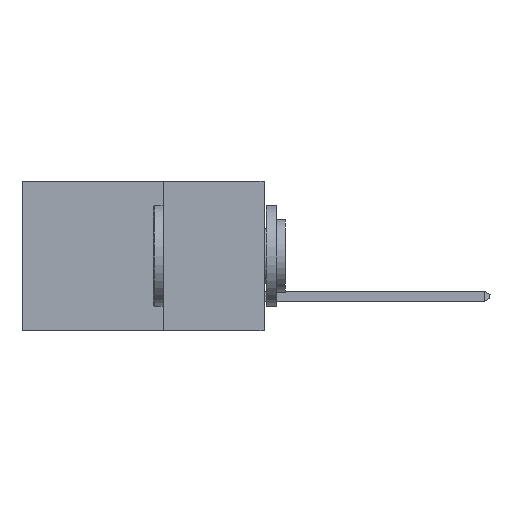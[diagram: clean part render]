
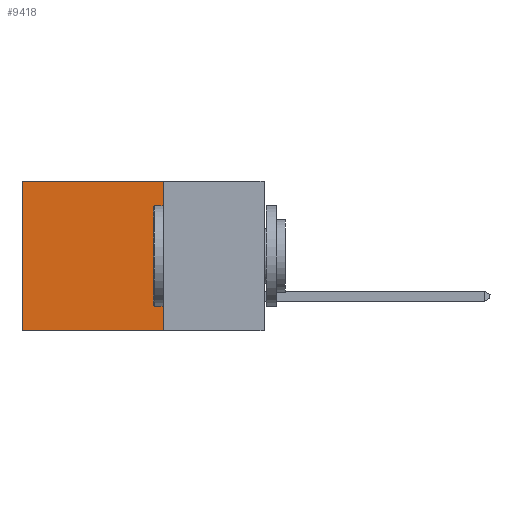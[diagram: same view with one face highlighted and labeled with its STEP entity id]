
A CAD part, left-side view. The second image highlights one B-rep face of the part: STEP entity #9418.
In plain terms, the highlighted planar face has unit normal (-1, 0, 0).
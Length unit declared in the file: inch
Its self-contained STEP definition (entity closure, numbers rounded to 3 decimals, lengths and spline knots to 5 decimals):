
#198 = LINE ( 'NONE', #7642, #2643 ) ;
#1241 = ORIENTED_EDGE ( 'NONE', *, *, #16333, .T. ) ;
#2643 = VECTOR ( 'NONE', #11825, 39.37008 ) ;
#2667 = DIRECTION ( 'NONE',  ( 1., 0., 0. ) ) ;
#2674 = CARTESIAN_POINT ( 'NONE',  ( 0.2615, 0.25, 0. ) ) ;
#3452 = CARTESIAN_POINT ( 'NONE',  ( 0.2615, 0.25, -0.37 ) ) ;
#3565 = DIRECTION ( 'NONE',  ( 0., 0., -1. ) ) ;
#3681 = VERTEX_POINT ( 'NONE', #11476 ) ;
#4218 = AXIS2_PLACEMENT_3D ( 'NONE', #10001, #2667, #5284 ) ;
#4469 = LINE ( 'NONE', #17436, #14723 ) ;
#5212 = LINE ( 'NONE', #3452, #6943 ) ;
#5284 = DIRECTION ( 'NONE',  ( 0., 0., -1. ) ) ;
#6100 = CARTESIAN_POINT ( 'NONE',  ( 0.2615, 0.25, 0. ) ) ;
#6922 = ORIENTED_EDGE ( 'NONE', *, *, #9946, .F. ) ;
#6943 = VECTOR ( 'NONE', #3565, 39.37008 ) ;
#7642 = CARTESIAN_POINT ( 'NONE',  ( 0.2615, 0.6, -0.37 ) ) ;
#9173 = DIRECTION ( 'NONE',  ( 0., 1., 0. ) ) ;
#9208 = VERTEX_POINT ( 'NONE', #16688 ) ;
#9418 = ADVANCED_FACE ( 'NONE', ( #15910 ), #17362, .F. ) ;
#9734 = VECTOR ( 'NONE', #9173, 39.37008 ) ;
#9946 = EDGE_CURVE ( 'NONE', #3681, #9208, #4469, .T. ) ;
#10001 = CARTESIAN_POINT ( 'NONE',  ( 0.2615, 0.25, -0.37 ) ) ;
#11476 = CARTESIAN_POINT ( 'NONE',  ( 0.2615, 0.25, -0.37 ) ) ;
#11498 = VERTEX_POINT ( 'NONE', #16389 ) ;
#11825 = DIRECTION ( 'NONE',  ( 0., 0., -1. ) ) ;
#13831 = EDGE_CURVE ( 'NONE', #15693, #3681, #5212, .T. ) ;
#14405 = ORIENTED_EDGE ( 'NONE', *, *, #13831, .F. ) ;
#14723 = VECTOR ( 'NONE', #16261, 39.37008 ) ;
#15693 = VERTEX_POINT ( 'NONE', #2674 ) ;
#15910 = FACE_OUTER_BOUND ( 'NONE', #17920, .T. ) ;
#16261 = DIRECTION ( 'NONE',  ( 0., 1., 0. ) ) ;
#16268 = LINE ( 'NONE', #6100, #9734 ) ;
#16311 = EDGE_CURVE ( 'NONE', #11498, #9208, #198, .T. ) ;
#16333 = EDGE_CURVE ( 'NONE', #15693, #11498, #16268, .T. ) ;
#16389 = CARTESIAN_POINT ( 'NONE',  ( 0.2615, 0.6, 0. ) ) ;
#16688 = CARTESIAN_POINT ( 'NONE',  ( 0.2615, 0.6, -0.37 ) ) ;
#17234 = ORIENTED_EDGE ( 'NONE', *, *, #16311, .T. ) ;
#17362 = PLANE ( 'NONE',  #4218 ) ;
#17436 = CARTESIAN_POINT ( 'NONE',  ( 0.2615, 0.25, -0.37 ) ) ;
#17920 = EDGE_LOOP ( 'NONE', ( #17234, #6922, #14405, #1241 ) ) ;
